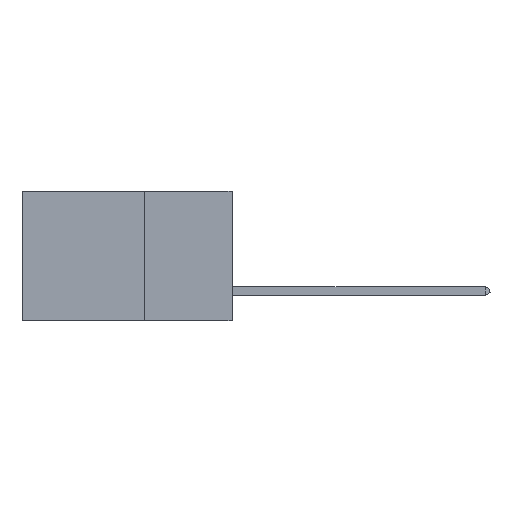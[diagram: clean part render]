
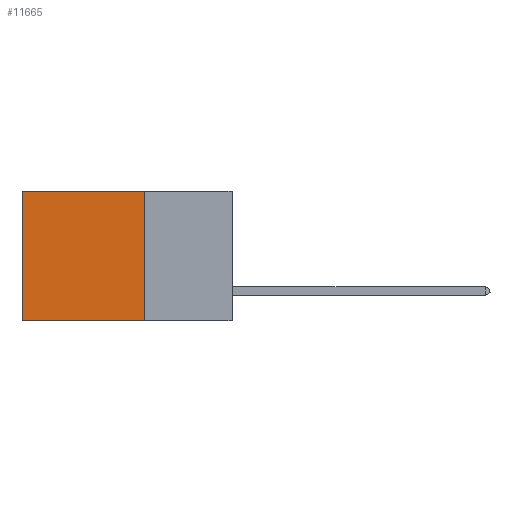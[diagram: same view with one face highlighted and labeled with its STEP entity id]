
A CAD part, left-side view. The second image highlights one B-rep face of the part: STEP entity #11665.
In plain terms, the highlighted planar face has unit normal (-1, 0, 0).
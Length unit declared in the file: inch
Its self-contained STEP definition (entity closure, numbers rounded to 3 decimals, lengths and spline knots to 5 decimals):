
#182 = EDGE_CURVE ( 'NONE', #10818, #12553, #5662, .T. ) ;
#487 = PLANE ( 'NONE',  #10666 ) ;
#562 = CARTESIAN_POINT ( 'NONE',  ( 0.2875, 0.6, -0.37 ) ) ;
#779 = EDGE_LOOP ( 'NONE', ( #11325, #15662, #21155, #13469 ) ) ;
#2255 = CARTESIAN_POINT ( 'NONE',  ( 0.2875, 0.6, 0. ) ) ;
#2930 = LINE ( 'NONE', #2255, #5168 ) ;
#3541 = VERTEX_POINT ( 'NONE', #3991 ) ;
#3991 = CARTESIAN_POINT ( 'NONE',  ( 0.2875, 0.6, 0. ) ) ;
#4242 = CARTESIAN_POINT ( 'NONE',  ( 0.2875, 0.25, 0. ) ) ;
#4835 = VECTOR ( 'NONE', #18201, 39.37008 ) ;
#5168 = VECTOR ( 'NONE', #22090, 39.37008 ) ;
#5595 = CARTESIAN_POINT ( 'NONE',  ( 0.2875, 0.25, 0. ) ) ;
#5662 = LINE ( 'NONE', #16541, #4835 ) ;
#7137 = LINE ( 'NONE', #19997, #22758 ) ;
#7768 = DIRECTION ( 'NONE',  ( 0., 0., -1. ) ) ;
#8479 = VECTOR ( 'NONE', #21853, 39.37008 ) ;
#9220 = CARTESIAN_POINT ( 'NONE',  ( 0.2875, 0.25, -0.37 ) ) ;
#9245 = EDGE_CURVE ( 'NONE', #3541, #12553, #2930, .T. ) ;
#10151 = LINE ( 'NONE', #5595, #8479 ) ;
#10372 = FACE_OUTER_BOUND ( 'NONE', #779, .T. ) ;
#10666 = AXIS2_PLACEMENT_3D ( 'NONE', #4242, #13047, #7768 ) ;
#10818 = VERTEX_POINT ( 'NONE', #9220 ) ;
#10955 = DIRECTION ( 'NONE',  ( 0., 0., -1. ) ) ;
#11325 = ORIENTED_EDGE ( 'NONE', *, *, #9245, .T. ) ;
#11665 = ADVANCED_FACE ( 'NONE', ( #10372 ), #487, .F. ) ;
#12553 = VERTEX_POINT ( 'NONE', #562 ) ;
#13047 = DIRECTION ( 'NONE',  ( 1., 0., 0. ) ) ;
#13397 = VERTEX_POINT ( 'NONE', #14525 ) ;
#13469 = ORIENTED_EDGE ( 'NONE', *, *, #15727, .T. ) ;
#14525 = CARTESIAN_POINT ( 'NONE',  ( 0.2875, 0.25, 0. ) ) ;
#15662 = ORIENTED_EDGE ( 'NONE', *, *, #182, .F. ) ;
#15727 = EDGE_CURVE ( 'NONE', #13397, #3541, #10151, .T. ) ;
#16541 = CARTESIAN_POINT ( 'NONE',  ( 0.2875, 0.25, -0.37 ) ) ;
#18201 = DIRECTION ( 'NONE',  ( 0., 1., 0. ) ) ;
#19997 = CARTESIAN_POINT ( 'NONE',  ( 0.2875, 0.25, 0. ) ) ;
#21155 = ORIENTED_EDGE ( 'NONE', *, *, #21527, .F. ) ;
#21527 = EDGE_CURVE ( 'NONE', #13397, #10818, #7137, .T. ) ;
#21853 = DIRECTION ( 'NONE',  ( 0., 1., 0. ) ) ;
#22090 = DIRECTION ( 'NONE',  ( 0., 0., -1. ) ) ;
#22758 = VECTOR ( 'NONE', #10955, 39.37008 ) ;
